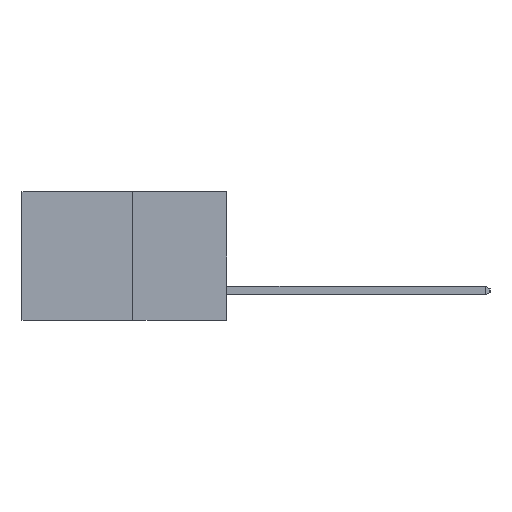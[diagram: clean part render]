
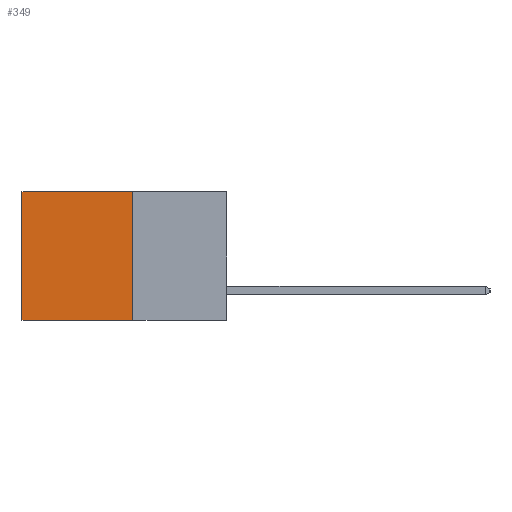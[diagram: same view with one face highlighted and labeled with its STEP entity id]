
A CAD part, left-side view. The second image highlights one B-rep face of the part: STEP entity #349.
In plain terms, the highlighted planar face has unit normal (-1, 0, 0).
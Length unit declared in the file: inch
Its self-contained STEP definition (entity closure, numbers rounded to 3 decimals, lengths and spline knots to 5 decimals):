
#349 = ADVANCED_FACE ( 'NONE', ( #5944 ), #6433, .F. ) ;
#615 = VERTEX_POINT ( 'NONE', #8073 ) ;
#682 = VECTOR ( 'NONE', #4451, 39.37008 ) ;
#751 = CARTESIAN_POINT ( 'NONE',  ( 0.277, 0.59, -0.37 ) ) ;
#905 = DIRECTION ( 'NONE',  ( 0., 1., 0. ) ) ;
#1922 = LINE ( 'NONE', #3121, #3518 ) ;
#1936 = DIRECTION ( 'NONE',  ( 0., 1., 0. ) ) ;
#2406 = EDGE_CURVE ( 'NONE', #615, #3074, #6930, .T. ) ;
#2420 = EDGE_CURVE ( 'NONE', #4880, #8225, #6333, .T. ) ;
#3074 = VERTEX_POINT ( 'NONE', #7140 ) ;
#3121 = CARTESIAN_POINT ( 'NONE',  ( 0.277, 0.59, -0.37 ) ) ;
#3303 = EDGE_CURVE ( 'NONE', #615, #4880, #4341, .T. ) ;
#3518 = VECTOR ( 'NONE', #8402, 39.37008 ) ;
#3743 = CARTESIAN_POINT ( 'NONE',  ( 0.277, 0.27, -0.37 ) ) ;
#4284 = ORIENTED_EDGE ( 'NONE', *, *, #8449, .T. ) ;
#4341 = LINE ( 'NONE', #4459, #682 ) ;
#4451 = DIRECTION ( 'NONE',  ( 0., 0., -1. ) ) ;
#4459 = CARTESIAN_POINT ( 'NONE',  ( 0.277, 0.27, -0.37 ) ) ;
#4553 = DIRECTION ( 'NONE',  ( 1., 0., 0. ) ) ;
#4573 = VECTOR ( 'NONE', #1936, 39.37008 ) ;
#4581 = DIRECTION ( 'NONE',  ( 0., 0., -1. ) ) ;
#4786 = VECTOR ( 'NONE', #905, 39.37008 ) ;
#4880 = VERTEX_POINT ( 'NONE', #6079 ) ;
#5000 = ORIENTED_EDGE ( 'NONE', *, *, #2406, .T. ) ;
#5944 = FACE_OUTER_BOUND ( 'NONE', #8614, .T. ) ;
#6079 = CARTESIAN_POINT ( 'NONE',  ( 0.277, 0.27, -0.37 ) ) ;
#6333 = LINE ( 'NONE', #3743, #4573 ) ;
#6433 = PLANE ( 'NONE',  #8502 ) ;
#6472 = ORIENTED_EDGE ( 'NONE', *, *, #2420, .F. ) ;
#6802 = ORIENTED_EDGE ( 'NONE', *, *, #3303, .F. ) ;
#6930 = LINE ( 'NONE', #8574, #4786 ) ;
#7063 = CARTESIAN_POINT ( 'NONE',  ( 0.277, 0.27, -0.37 ) ) ;
#7140 = CARTESIAN_POINT ( 'NONE',  ( 0.277, 0.59, 0. ) ) ;
#8073 = CARTESIAN_POINT ( 'NONE',  ( 0.277, 0.27, 0. ) ) ;
#8225 = VERTEX_POINT ( 'NONE', #751 ) ;
#8402 = DIRECTION ( 'NONE',  ( 0., 0., -1. ) ) ;
#8449 = EDGE_CURVE ( 'NONE', #3074, #8225, #1922, .T. ) ;
#8502 = AXIS2_PLACEMENT_3D ( 'NONE', #7063, #4553, #4581 ) ;
#8574 = CARTESIAN_POINT ( 'NONE',  ( 0.277, 0.27, 0. ) ) ;
#8614 = EDGE_LOOP ( 'NONE', ( #4284, #6472, #6802, #5000 ) ) ;
